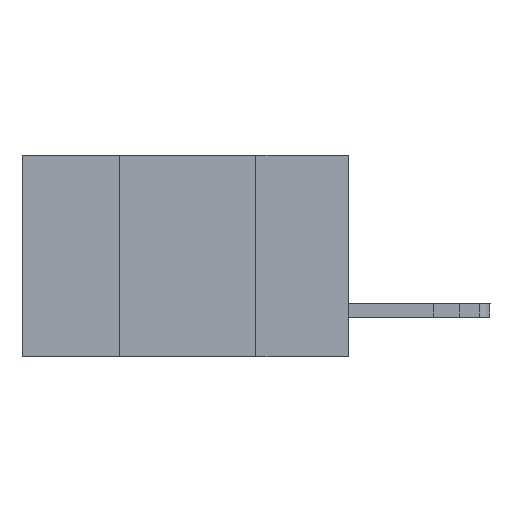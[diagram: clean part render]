
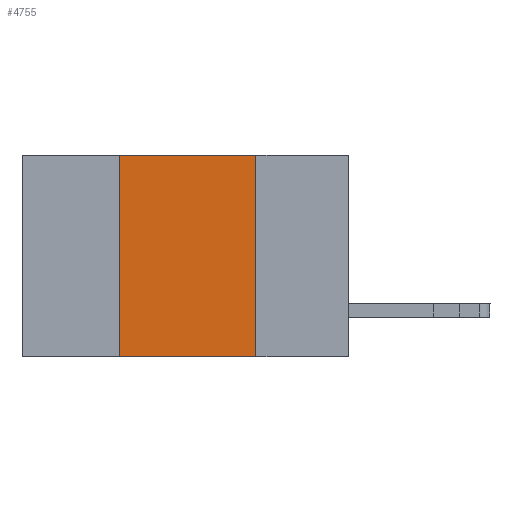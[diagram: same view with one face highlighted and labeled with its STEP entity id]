
A CAD part, left-side view. The second image highlights one B-rep face of the part: STEP entity #4755.
In plain terms, the highlighted planar face has unit normal (-1, 0, 0).
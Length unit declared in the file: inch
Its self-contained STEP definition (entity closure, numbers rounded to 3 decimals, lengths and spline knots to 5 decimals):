
#119 = CARTESIAN_POINT ( 'NONE',  ( 0., 0.17, -0.37 ) ) ;
#154 = VECTOR ( 'NONE', #9320, 39.37008 ) ;
#253 = EDGE_CURVE ( 'NONE', #1953, #8239, #8071, .T. ) ;
#919 = CARTESIAN_POINT ( 'NONE',  ( 0., 0.6, -0.37 ) ) ;
#1037 = LINE ( 'NONE', #119, #154 ) ;
#1953 = VERTEX_POINT ( 'NONE', #11621 ) ;
#2082 = CARTESIAN_POINT ( 'NONE',  ( 0., 0.42, -0.37 ) ) ;
#2098 = FACE_OUTER_BOUND ( 'NONE', #10686, .T. ) ;
#2154 = CARTESIAN_POINT ( 'NONE',  ( 0., 0.6, 0. ) ) ;
#2847 = DIRECTION ( 'NONE',  ( 0., -1., 0. ) ) ;
#3048 = LINE ( 'NONE', #2154, #7677 ) ;
#3051 = CARTESIAN_POINT ( 'NONE',  ( 0., 0.42, 0. ) ) ;
#3128 = ORIENTED_EDGE ( 'NONE', *, *, #4753, .F. ) ;
#3907 = CARTESIAN_POINT ( 'NONE',  ( 0., 0.6, 0. ) ) ;
#4753 = EDGE_CURVE ( 'NONE', #5913, #5092, #3048, .T. ) ;
#4755 = ADVANCED_FACE ( 'NONE', ( #2098 ), #5689, .F. ) ;
#5092 = VERTEX_POINT ( 'NONE', #8547 ) ;
#5385 = EDGE_CURVE ( 'NONE', #5092, #8239, #1037, .T. ) ;
#5598 = AXIS2_PLACEMENT_3D ( 'NONE', #3907, #11130, #5751 ) ;
#5683 = VECTOR ( 'NONE', #10999, 39.37008 ) ;
#5689 = PLANE ( 'NONE',  #5598 ) ;
#5714 = ORIENTED_EDGE ( 'NONE', *, *, #5385, .F. ) ;
#5751 = DIRECTION ( 'NONE',  ( 0., 0., -1. ) ) ;
#5913 = VERTEX_POINT ( 'NONE', #3051 ) ;
#7563 = LINE ( 'NONE', #2082, #5683 ) ;
#7677 = VECTOR ( 'NONE', #9424, 39.37008 ) ;
#8004 = EDGE_CURVE ( 'NONE', #1953, #5913, #7563, .T. ) ;
#8071 = LINE ( 'NONE', #919, #9494 ) ;
#8239 = VERTEX_POINT ( 'NONE', #9410 ) ;
#8371 = ORIENTED_EDGE ( 'NONE', *, *, #8004, .F. ) ;
#8547 = CARTESIAN_POINT ( 'NONE',  ( 0., 0.17, 0. ) ) ;
#9320 = DIRECTION ( 'NONE',  ( 0., 0., -1. ) ) ;
#9410 = CARTESIAN_POINT ( 'NONE',  ( 0., 0.17, -0.37 ) ) ;
#9424 = DIRECTION ( 'NONE',  ( 0., -1., 0. ) ) ;
#9494 = VECTOR ( 'NONE', #2847, 39.37008 ) ;
#9636 = ORIENTED_EDGE ( 'NONE', *, *, #253, .T. ) ;
#10686 = EDGE_LOOP ( 'NONE', ( #5714, #3128, #8371, #9636 ) ) ;
#10999 = DIRECTION ( 'NONE',  ( 0., 0., 1. ) ) ;
#11130 = DIRECTION ( 'NONE',  ( 1., 0., 0. ) ) ;
#11621 = CARTESIAN_POINT ( 'NONE',  ( 0., 0.42, -0.37 ) ) ;
